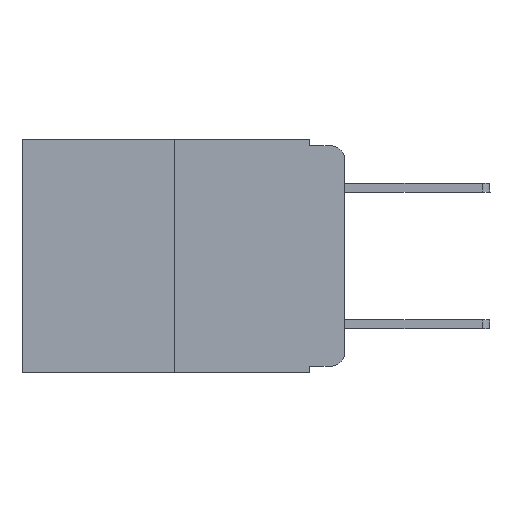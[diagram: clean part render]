
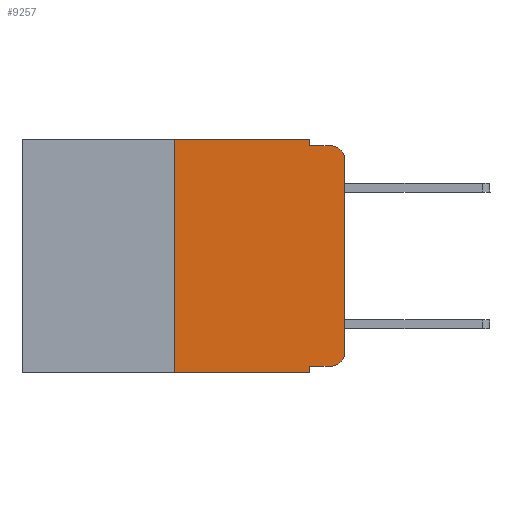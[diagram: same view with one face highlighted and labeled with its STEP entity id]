
A CAD part, left-side view. The second image highlights one B-rep face of the part: STEP entity #9257.
In plain terms, the highlighted planar face has unit normal (-1, 0, 0).
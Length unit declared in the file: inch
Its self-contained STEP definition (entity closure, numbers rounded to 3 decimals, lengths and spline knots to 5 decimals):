
#510 = CARTESIAN_POINT ( 'NONE',  ( 0., 0.25, 0. ) ) ;
#526 = CARTESIAN_POINT ( 'NONE',  ( 0., 0.473, 0. ) ) ;
#1272 = EDGE_CURVE ( 'NONE', #7042, #11952, #20256, .T. ) ;
#1327 = DIRECTION ( 'NONE',  ( 0., 0., 1. ) ) ;
#1535 = AXIS2_PLACEMENT_3D ( 'NONE', #22015, #13811, #20386 ) ;
#1577 = CARTESIAN_POINT ( 'NONE',  ( 0., 0.051, 0. ) ) ;
#1583 = VECTOR ( 'NONE', #16023, 39.37008 ) ;
#1667 = VECTOR ( 'NONE', #4875, 39.37008 ) ;
#2448 = CARTESIAN_POINT ( 'NONE',  ( 0., 0.051, -0.01 ) ) ;
#2817 = LINE ( 'NONE', #4743, #1667 ) ;
#2896 = AXIS2_PLACEMENT_3D ( 'NONE', #526, #17230, #17107 ) ;
#2900 = CARTESIAN_POINT ( 'NONE',  ( 0., 0.051, 0. ) ) ;
#3046 = EDGE_LOOP ( 'NONE', ( #4129, #18292, #18449, #26141, #21878, #24232, #21989, #23135, #22922, #3887 ) ) ;
#3459 = VECTOR ( 'NONE', #19619, 39.37008 ) ;
#3693 = CARTESIAN_POINT ( 'NONE',  ( 0., 0.02, -0.03 ) ) ;
#3754 = VECTOR ( 'NONE', #9500, 39.37008 ) ;
#3849 = CIRCLE ( 'NONE', #4706, 0.02 ) ;
#3887 = ORIENTED_EDGE ( 'NONE', *, *, #21751, .T. ) ;
#4129 = ORIENTED_EDGE ( 'NONE', *, *, #26309, .T. ) ;
#4238 = EDGE_CURVE ( 'NONE', #22041, #14698, #23845, .T. ) ;
#4706 = AXIS2_PLACEMENT_3D ( 'NONE', #3693, #11609, #20254 ) ;
#4743 = CARTESIAN_POINT ( 'NONE',  ( 0., 0.051, 0. ) ) ;
#4875 = DIRECTION ( 'NONE',  ( 0., 0., -1. ) ) ;
#5408 = DIRECTION ( 'NONE',  ( 0., 0., -1. ) ) ;
#7042 = VERTEX_POINT ( 'NONE', #21559 ) ;
#7388 = LINE ( 'NONE', #7807, #1583 ) ;
#7512 = CARTESIAN_POINT ( 'NONE',  ( 0., 0.051, -0.333 ) ) ;
#7573 = CARTESIAN_POINT ( 'NONE',  ( 0., 0.25, 0. ) ) ;
#7613 = CARTESIAN_POINT ( 'NONE',  ( 0., 0., 0. ) ) ;
#7629 = DIRECTION ( 'NONE',  ( 0., -1., 0. ) ) ;
#7807 = CARTESIAN_POINT ( 'NONE',  ( 0., 0.051, -0.333 ) ) ;
#7995 = VERTEX_POINT ( 'NONE', #2448 ) ;
#8625 = CARTESIAN_POINT ( 'NONE',  ( 0., 0.051, -0.343 ) ) ;
#8684 = VECTOR ( 'NONE', #12171, 39.37008 ) ;
#9044 = EDGE_CURVE ( 'NONE', #21757, #14938, #7388, .T. ) ;
#9257 = ADVANCED_FACE ( 'NONE', ( #15309 ), #23254, .F. ) ;
#9500 = DIRECTION ( 'NONE',  ( 0., 0., 1. ) ) ;
#9993 = CARTESIAN_POINT ( 'NONE',  ( 0., 0.473, -0.343 ) ) ;
#10988 = EDGE_CURVE ( 'NONE', #14698, #7995, #2817, .T. ) ;
#11609 = DIRECTION ( 'NONE',  ( -1., 0., 0. ) ) ;
#11952 = VERTEX_POINT ( 'NONE', #8625 ) ;
#12152 = LINE ( 'NONE', #18180, #22344 ) ;
#12171 = DIRECTION ( 'NONE',  ( 0., -1., 0. ) ) ;
#13811 = DIRECTION ( 'NONE',  ( -1., 0., 0. ) ) ;
#14217 = CARTESIAN_POINT ( 'NONE',  ( 0., 0., -0.03 ) ) ;
#14698 = VERTEX_POINT ( 'NONE', #2900 ) ;
#14938 = VERTEX_POINT ( 'NONE', #23280 ) ;
#15309 = FACE_OUTER_BOUND ( 'NONE', #3046, .T. ) ;
#15642 = VECTOR ( 'NONE', #1327, 39.37008 ) ;
#15811 = VECTOR ( 'NONE', #5408, 39.37008 ) ;
#16023 = DIRECTION ( 'NONE',  ( 0., -1., 0. ) ) ;
#16595 = EDGE_CURVE ( 'NONE', #7995, #24724, #12152, .T. ) ;
#17061 = EDGE_CURVE ( 'NONE', #21757, #11952, #22506, .T. ) ;
#17107 = DIRECTION ( 'NONE',  ( 0., 0., -1. ) ) ;
#17230 = DIRECTION ( 'NONE',  ( 1., 0., 0. ) ) ;
#17895 = LINE ( 'NONE', #7613, #15642 ) ;
#18180 = CARTESIAN_POINT ( 'NONE',  ( 0., 0.051, -0.01 ) ) ;
#18292 = ORIENTED_EDGE ( 'NONE', *, *, #25774, .T. ) ;
#18449 = ORIENTED_EDGE ( 'NONE', *, *, #16595, .F. ) ;
#19619 = DIRECTION ( 'NONE',  ( 0., -1., 0. ) ) ;
#20254 = DIRECTION ( 'NONE',  ( 0., 0., -1. ) ) ;
#20256 = LINE ( 'NONE', #9993, #8684 ) ;
#20386 = DIRECTION ( 'NONE',  ( 0., 0., -1. ) ) ;
#21517 = CARTESIAN_POINT ( 'NONE',  ( 0., 0.473, 0. ) ) ;
#21559 = CARTESIAN_POINT ( 'NONE',  ( 0., 0.25, -0.343 ) ) ;
#21751 = EDGE_CURVE ( 'NONE', #14938, #26948, #26430, .T. ) ;
#21757 = VERTEX_POINT ( 'NONE', #7512 ) ;
#21878 = ORIENTED_EDGE ( 'NONE', *, *, #4238, .F. ) ;
#21989 = ORIENTED_EDGE ( 'NONE', *, *, #1272, .T. ) ;
#22015 = CARTESIAN_POINT ( 'NONE',  ( 0., 0.02, -0.313 ) ) ;
#22041 = VERTEX_POINT ( 'NONE', #510 ) ;
#22344 = VECTOR ( 'NONE', #7629, 39.37008 ) ;
#22506 = LINE ( 'NONE', #1577, #15811 ) ;
#22523 = EDGE_CURVE ( 'NONE', #7042, #22041, #24004, .T. ) ;
#22763 = CARTESIAN_POINT ( 'NONE',  ( 0., 0., -0.313 ) ) ;
#22922 = ORIENTED_EDGE ( 'NONE', *, *, #9044, .T. ) ;
#23135 = ORIENTED_EDGE ( 'NONE', *, *, #17061, .F. ) ;
#23235 = CARTESIAN_POINT ( 'NONE',  ( 0., 0.02, -0.01 ) ) ;
#23254 = PLANE ( 'NONE',  #2896 ) ;
#23280 = CARTESIAN_POINT ( 'NONE',  ( 0., 0.02, -0.333 ) ) ;
#23845 = LINE ( 'NONE', #21517, #3459 ) ;
#24004 = LINE ( 'NONE', #7573, #3754 ) ;
#24232 = ORIENTED_EDGE ( 'NONE', *, *, #22523, .F. ) ;
#24542 = VERTEX_POINT ( 'NONE', #14217 ) ;
#24724 = VERTEX_POINT ( 'NONE', #23235 ) ;
#25774 = EDGE_CURVE ( 'NONE', #24542, #24724, #3849, .T. ) ;
#26141 = ORIENTED_EDGE ( 'NONE', *, *, #10988, .F. ) ;
#26309 = EDGE_CURVE ( 'NONE', #26948, #24542, #17895, .T. ) ;
#26430 = CIRCLE ( 'NONE', #1535, 0.02 ) ;
#26948 = VERTEX_POINT ( 'NONE', #22763 ) ;
